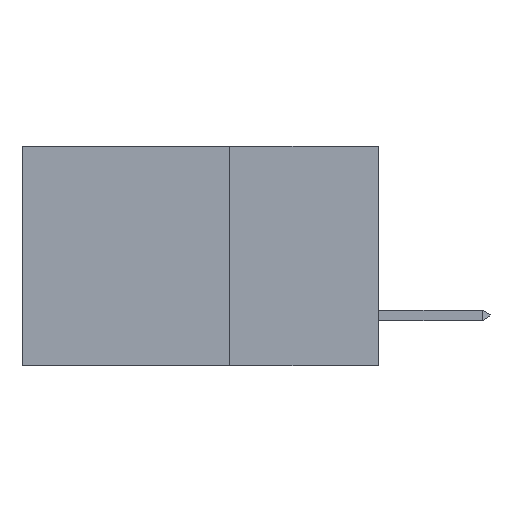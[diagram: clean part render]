
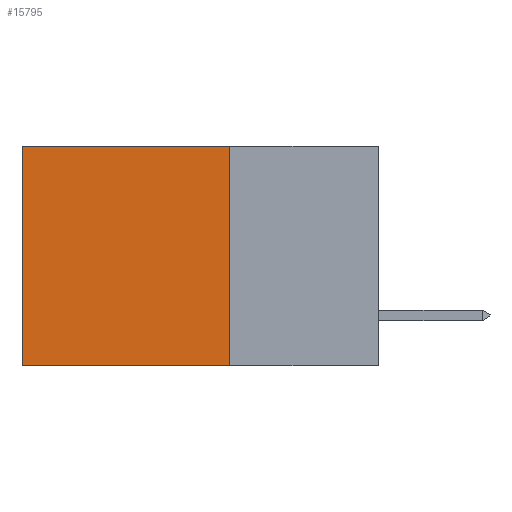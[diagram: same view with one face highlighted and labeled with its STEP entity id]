
A CAD part, left-side view. The second image highlights one B-rep face of the part: STEP entity #15795.
In plain terms, the highlighted planar face has unit normal (-1, 0, 0).
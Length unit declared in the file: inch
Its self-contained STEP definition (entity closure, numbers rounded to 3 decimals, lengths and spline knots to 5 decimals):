
#630 = CARTESIAN_POINT ( 'NONE',  ( 0.2615, 0.6, -0.37 ) ) ;
#1926 = ORIENTED_EDGE ( 'NONE', *, *, #2489, .T. ) ;
#2416 = CARTESIAN_POINT ( 'NONE',  ( 0.2615, 0.25, -0.37 ) ) ;
#2489 = EDGE_CURVE ( 'NONE', #15624, #4042, #2895, .T. ) ;
#2895 = LINE ( 'NONE', #6668, #15645 ) ;
#3284 = ORIENTED_EDGE ( 'NONE', *, *, #6930, .F. ) ;
#3759 = DIRECTION ( 'NONE',  ( 0., 0., -1. ) ) ;
#4042 = VERTEX_POINT ( 'NONE', #12190 ) ;
#4406 = CARTESIAN_POINT ( 'NONE',  ( 0.2615, 0.25, -0.37 ) ) ;
#4568 = VECTOR ( 'NONE', #5367, 39.37008 ) ;
#4619 = VECTOR ( 'NONE', #3759, 39.37008 ) ;
#4665 = DIRECTION ( 'NONE',  ( 1., 0., 0. ) ) ;
#4689 = ORIENTED_EDGE ( 'NONE', *, *, #14571, .F. ) ;
#5230 = CARTESIAN_POINT ( 'NONE',  ( 0.2615, 0.6, -0.37 ) ) ;
#5367 = DIRECTION ( 'NONE',  ( 0., 0., -1. ) ) ;
#6668 = CARTESIAN_POINT ( 'NONE',  ( 0.2615, 0.25, 0. ) ) ;
#6836 = CARTESIAN_POINT ( 'NONE',  ( 0.2615, 0.25, -0.37 ) ) ;
#6930 = EDGE_CURVE ( 'NONE', #10649, #10687, #10441, .T. ) ;
#7081 = VECTOR ( 'NONE', #9243, 39.37008 ) ;
#8094 = LINE ( 'NONE', #630, #4568 ) ;
#8276 = DIRECTION ( 'NONE',  ( 0., 0., -1. ) ) ;
#8424 = CARTESIAN_POINT ( 'NONE',  ( 0.2615, 0.25, 0. ) ) ;
#8837 = ORIENTED_EDGE ( 'NONE', *, *, #11253, .T. ) ;
#9243 = DIRECTION ( 'NONE',  ( 0., 1., 0. ) ) ;
#10441 = LINE ( 'NONE', #4406, #7081 ) ;
#10649 = VERTEX_POINT ( 'NONE', #11187 ) ;
#10687 = VERTEX_POINT ( 'NONE', #5230 ) ;
#11066 = AXIS2_PLACEMENT_3D ( 'NONE', #6836, #4665, #8276 ) ;
#11187 = CARTESIAN_POINT ( 'NONE',  ( 0.2615, 0.25, -0.37 ) ) ;
#11253 = EDGE_CURVE ( 'NONE', #4042, #10687, #8094, .T. ) ;
#12088 = EDGE_LOOP ( 'NONE', ( #8837, #3284, #4689, #1926 ) ) ;
#12190 = CARTESIAN_POINT ( 'NONE',  ( 0.2615, 0.6, 0. ) ) ;
#13349 = FACE_OUTER_BOUND ( 'NONE', #12088, .T. ) ;
#13683 = DIRECTION ( 'NONE',  ( 0., 1., 0. ) ) ;
#14571 = EDGE_CURVE ( 'NONE', #15624, #10649, #14787, .T. ) ;
#14787 = LINE ( 'NONE', #2416, #4619 ) ;
#15613 = PLANE ( 'NONE',  #11066 ) ;
#15624 = VERTEX_POINT ( 'NONE', #8424 ) ;
#15645 = VECTOR ( 'NONE', #13683, 39.37008 ) ;
#15795 = ADVANCED_FACE ( 'NONE', ( #13349 ), #15613, .F. ) ;
